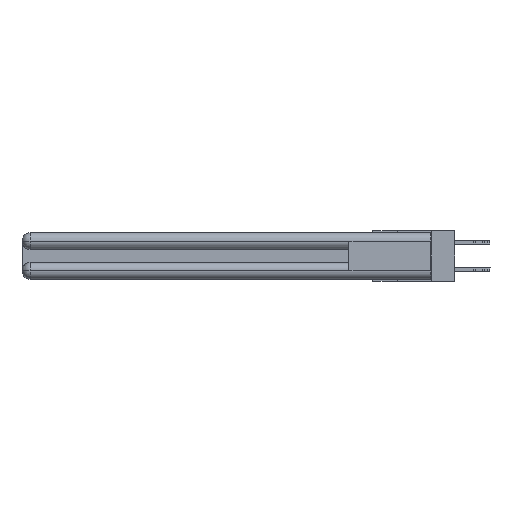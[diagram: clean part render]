
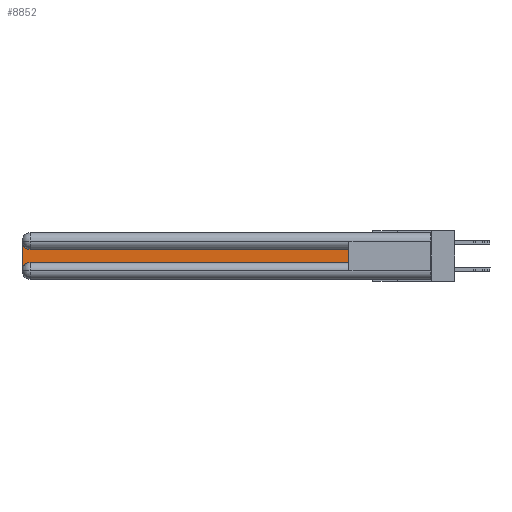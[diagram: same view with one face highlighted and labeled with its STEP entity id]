
A CAD part, left-side view. The second image highlights one B-rep face of the part: STEP entity #8852.
In plain terms, the highlighted planar face has unit normal (-1, 0, 0).
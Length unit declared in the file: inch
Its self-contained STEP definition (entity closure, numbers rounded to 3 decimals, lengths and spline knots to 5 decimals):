
#525 = VECTOR ( 'NONE', #6533, 39.37008 ) ;
#744 = EDGE_LOOP ( 'NONE', ( #2803, #8592, #19041, #10390, #7689, #16909 ) ) ;
#1710 = CARTESIAN_POINT ( 'NONE',  ( 0.075, 2.94, -0.2775 ) ) ;
#2281 = CARTESIAN_POINT ( 'NONE',  ( 0.075, 3., -0.1225 ) ) ;
#2357 = DIRECTION ( 'NONE',  ( 1., 0., 0. ) ) ;
#2803 = ORIENTED_EDGE ( 'NONE', *, *, #25174, .T. ) ;
#3838 = CARTESIAN_POINT ( 'NONE',  ( 0.075, 2.94, -0.1225 ) ) ;
#4177 = FACE_OUTER_BOUND ( 'NONE', #744, .T. ) ;
#4456 = DIRECTION ( 'NONE',  ( 0., 0., -1. ) ) ;
#4882 = VERTEX_POINT ( 'NONE', #3838 ) ;
#6138 = EDGE_CURVE ( 'NONE', #24580, #13915, #10809, .T. ) ;
#6207 = CARTESIAN_POINT ( 'NONE',  ( 0.075, 0.6, -0.1225 ) ) ;
#6533 = DIRECTION ( 'NONE',  ( 0., 0., 1. ) ) ;
#7076 = VECTOR ( 'NONE', #12210, 39.37008 ) ;
#7455 = AXIS2_PLACEMENT_3D ( 'NONE', #1710, #8155, #23197 ) ;
#7689 = ORIENTED_EDGE ( 'NONE', *, *, #6138, .T. ) ;
#7871 = EDGE_CURVE ( 'NONE', #13915, #22235, #9705, .T. ) ;
#8155 = DIRECTION ( 'NONE',  ( 1., 0., 0. ) ) ;
#8592 = ORIENTED_EDGE ( 'NONE', *, *, #25772, .T. ) ;
#8852 = ADVANCED_FACE ( 'NONE', ( #4177 ), #17582, .F. ) ;
#9055 = CARTESIAN_POINT ( 'NONE',  ( 0.075, 0.6, -0.1225 ) ) ;
#9705 = LINE ( 'NONE', #15218, #525 ) ;
#10390 = ORIENTED_EDGE ( 'NONE', *, *, #17692, .T. ) ;
#10809 = LINE ( 'NONE', #27631, #7076 ) ;
#11107 = CARTESIAN_POINT ( 'NONE',  ( 0.075, 2.94, -0.0625 ) ) ;
#11523 = CARTESIAN_POINT ( 'NONE',  ( 0.075, 0.6, -0.2175 ) ) ;
#11692 = CARTESIAN_POINT ( 'NONE',  ( 0.075, 3., -0.0625 ) ) ;
#12210 = DIRECTION ( 'NONE',  ( 0., -1., 0. ) ) ;
#13908 = VERTEX_POINT ( 'NONE', #19728 ) ;
#13915 = VERTEX_POINT ( 'NONE', #11523 ) ;
#13948 = DIRECTION ( 'NONE',  ( 0., 0., -1. ) ) ;
#14849 = EDGE_CURVE ( 'NONE', #16821, #13908, #27202, .T. ) ;
#15218 = CARTESIAN_POINT ( 'NONE',  ( 0.075, 0.6, -0.2175 ) ) ;
#16316 = VECTOR ( 'NONE', #13948, 39.37008 ) ;
#16821 = VERTEX_POINT ( 'NONE', #11692 ) ;
#16861 = CARTESIAN_POINT ( 'NONE',  ( 0.075, 2.94, -0.2175 ) ) ;
#16909 = ORIENTED_EDGE ( 'NONE', *, *, #7871, .T. ) ;
#17480 = DIRECTION ( 'NONE',  ( 1., 0., 0. ) ) ;
#17582 = PLANE ( 'NONE',  #26451 ) ;
#17651 = DIRECTION ( 'NONE',  ( 0., 0., -1. ) ) ;
#17692 = EDGE_CURVE ( 'NONE', #13908, #24580, #24223, .T. ) ;
#19041 = ORIENTED_EDGE ( 'NONE', *, *, #14849, .T. ) ;
#19728 = CARTESIAN_POINT ( 'NONE',  ( 0.075, 3., -0.2775 ) ) ;
#20645 = CARTESIAN_POINT ( 'NONE',  ( 0.075, 3., -0.2175 ) ) ;
#21159 = LINE ( 'NONE', #6207, #25200 ) ;
#21301 = DIRECTION ( 'NONE',  ( 0., 1., 0. ) ) ;
#22235 = VERTEX_POINT ( 'NONE', #9055 ) ;
#23197 = DIRECTION ( 'NONE',  ( 0., 0., -1. ) ) ;
#23917 = AXIS2_PLACEMENT_3D ( 'NONE', #11107, #2357, #17651 ) ;
#24223 = CIRCLE ( 'NONE', #7455, 0.06 ) ;
#24580 = VERTEX_POINT ( 'NONE', #16861 ) ;
#25174 = EDGE_CURVE ( 'NONE', #22235, #4882, #21159, .T. ) ;
#25200 = VECTOR ( 'NONE', #21301, 39.37008 ) ;
#25772 = EDGE_CURVE ( 'NONE', #4882, #16821, #27572, .T. ) ;
#26451 = AXIS2_PLACEMENT_3D ( 'NONE', #2281, #17480, #4456 ) ;
#27202 = LINE ( 'NONE', #20645, #16316 ) ;
#27572 = CIRCLE ( 'NONE', #23917, 0.06 ) ;
#27631 = CARTESIAN_POINT ( 'NONE',  ( 0.075, 0.6, -0.2175 ) ) ;
